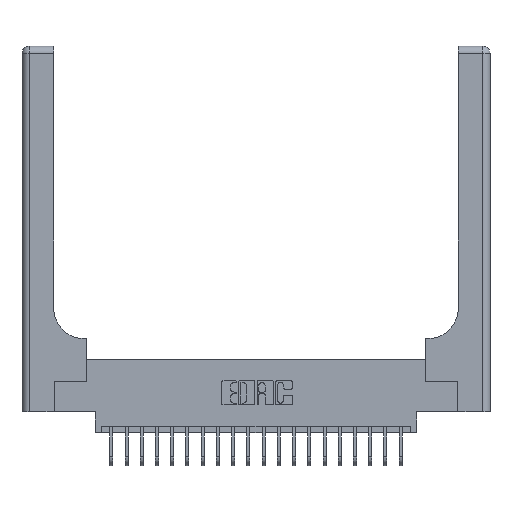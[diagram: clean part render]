
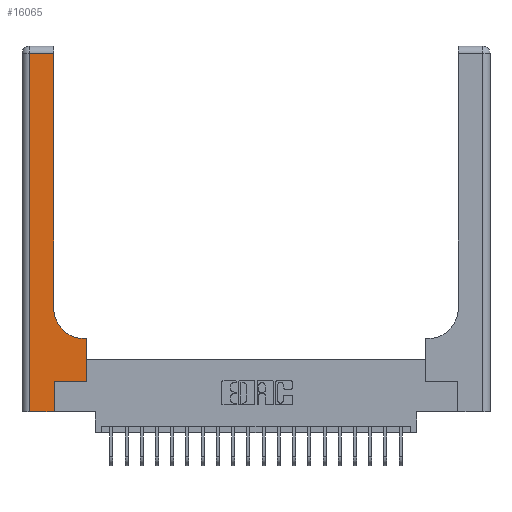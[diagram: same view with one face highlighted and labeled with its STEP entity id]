
A CAD part, top view. The second image highlights one B-rep face of the part: STEP entity #16065.
In plain terms, the highlighted planar face has unit normal (0, 0, 1).
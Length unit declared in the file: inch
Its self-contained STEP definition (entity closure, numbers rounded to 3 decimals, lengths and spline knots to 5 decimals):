
#262 = ORIENTED_EDGE ( 'NONE', *, *, #10968, .T. ) ;
#756 = ORIENTED_EDGE ( 'NONE', *, *, #4540, .T. ) ;
#783 = CARTESIAN_POINT ( 'NONE',  ( 0.528, 0.25, 0.37 ) ) ;
#866 = EDGE_CURVE ( 'NONE', #3148, #17993, #5105, .T. ) ;
#1039 = CARTESIAN_POINT ( 'NONE',  ( 0.265, 0.25, 0.37 ) ) ;
#1550 = VERTEX_POINT ( 'NONE', #18192 ) ;
#2073 = CARTESIAN_POINT ( 'NONE',  ( 0.51, 0.85, 0.37 ) ) ;
#2515 = AXIS2_PLACEMENT_3D ( 'NONE', #2073, #13334, #3703 ) ;
#2525 = CARTESIAN_POINT ( 'NONE',  ( 0.26, 0.6, 0.37 ) ) ;
#2943 = DIRECTION ( 'NONE',  ( -1., 0., 0. ) ) ;
#3007 = AXIS2_PLACEMENT_3D ( 'NONE', #17325, #12579, #2943 ) ;
#3048 = ORIENTED_EDGE ( 'NONE', *, *, #19050, .T. ) ;
#3148 = VERTEX_POINT ( 'NONE', #5501 ) ;
#3211 = EDGE_CURVE ( 'NONE', #4717, #1550, #7536, .T. ) ;
#3476 = VECTOR ( 'NONE', #15523, 39.37008 ) ;
#3703 = DIRECTION ( 'NONE',  ( 1., 0., 0. ) ) ;
#4015 = CARTESIAN_POINT ( 'NONE',  ( 0., 2.94, 0.37 ) ) ;
#4189 = CARTESIAN_POINT ( 'NONE',  ( 0.26, 3., 0.37 ) ) ;
#4418 = CARTESIAN_POINT ( 'NONE',  ( 0.265, 0., 0.37 ) ) ;
#4540 = EDGE_CURVE ( 'NONE', #6452, #16819, #16976, .T. ) ;
#4542 = CARTESIAN_POINT ( 'NONE',  ( 0.26, 2.94, 0.37 ) ) ;
#4717 = VERTEX_POINT ( 'NONE', #4542 ) ;
#5105 = LINE ( 'NONE', #16107, #17397 ) ;
#5501 = CARTESIAN_POINT ( 'NONE',  ( 0.06, 0., 0.37 ) ) ;
#5580 = ORIENTED_EDGE ( 'NONE', *, *, #14114, .T. ) ;
#5660 = VERTEX_POINT ( 'NONE', #17968 ) ;
#5806 = DIRECTION ( 'NONE',  ( 0., 1., 0. ) ) ;
#5862 = LINE ( 'NONE', #2525, #10161 ) ;
#5898 = CARTESIAN_POINT ( 'NONE',  ( 0.265, 0.25, 0.37 ) ) ;
#6035 = DIRECTION ( 'NONE',  ( 0., 1., 0. ) ) ;
#6452 = VERTEX_POINT ( 'NONE', #7565 ) ;
#6500 = DIRECTION ( 'NONE',  ( 1., 0., 0. ) ) ;
#7536 = LINE ( 'NONE', #4015, #14569 ) ;
#7565 = CARTESIAN_POINT ( 'NONE',  ( 0.528, 0.25, 0.37 ) ) ;
#7762 = LINE ( 'NONE', #5898, #3476 ) ;
#7835 = CARTESIAN_POINT ( 'NONE',  ( 0.26, 0.85, 0.37 ) ) ;
#8107 = CARTESIAN_POINT ( 'NONE',  ( 0.06, 3., 0.37 ) ) ;
#8207 = EDGE_CURVE ( 'NONE', #5660, #9135, #14369, .T. ) ;
#8454 = EDGE_CURVE ( 'NONE', #9135, #4717, #13604, .T. ) ;
#8461 = VECTOR ( 'NONE', #19999, 39.37008 ) ;
#9135 = VERTEX_POINT ( 'NONE', #7835 ) ;
#9410 = VECTOR ( 'NONE', #14565, 39.37008 ) ;
#9501 = CARTESIAN_POINT ( 'NONE',  ( 0.265, 0., 0.37 ) ) ;
#9694 = CARTESIAN_POINT ( 'NONE',  ( 0.528, 0.6, 0.37 ) ) ;
#10161 = VECTOR ( 'NONE', #15399, 39.37008 ) ;
#10968 = EDGE_CURVE ( 'NONE', #17200, #6452, #7762, .T. ) ;
#10985 = PLANE ( 'NONE',  #3007 ) ;
#11021 = EDGE_CURVE ( 'NONE', #17993, #17200, #19517, .T. ) ;
#11047 = VECTOR ( 'NONE', #6035, 39.37008 ) ;
#11612 = ORIENTED_EDGE ( 'NONE', *, *, #866, .T. ) ;
#12579 = DIRECTION ( 'NONE',  ( 0., 0., -1. ) ) ;
#12823 = FACE_OUTER_BOUND ( 'NONE', #16762, .T. ) ;
#13334 = DIRECTION ( 'NONE',  ( 0., 0., -1. ) ) ;
#13604 = LINE ( 'NONE', #4189, #17332 ) ;
#13672 = LINE ( 'NONE', #8107, #9410 ) ;
#14114 = EDGE_CURVE ( 'NONE', #16819, #5660, #5862, .T. ) ;
#14369 = CIRCLE ( 'NONE', #2515, 0.25 ) ;
#14565 = DIRECTION ( 'NONE',  ( 0., -1., 0. ) ) ;
#14569 = VECTOR ( 'NONE', #20034, 39.37008 ) ;
#15380 = ORIENTED_EDGE ( 'NONE', *, *, #8454, .T. ) ;
#15399 = DIRECTION ( 'NONE',  ( -1., 0., 0. ) ) ;
#15523 = DIRECTION ( 'NONE',  ( 1., 0., 0. ) ) ;
#16065 = ADVANCED_FACE ( 'NONE', ( #12823 ), #10985, .F. ) ;
#16107 = CARTESIAN_POINT ( 'NONE',  ( 0., 0., 0.37 ) ) ;
#16373 = ORIENTED_EDGE ( 'NONE', *, *, #11021, .T. ) ;
#16762 = EDGE_LOOP ( 'NONE', ( #15380, #19595, #3048, #11612, #16373, #262, #756, #5580, #18374 ) ) ;
#16819 = VERTEX_POINT ( 'NONE', #9694 ) ;
#16976 = LINE ( 'NONE', #783, #8461 ) ;
#17200 = VERTEX_POINT ( 'NONE', #1039 ) ;
#17325 = CARTESIAN_POINT ( 'NONE',  ( 0., 3., 0.37 ) ) ;
#17332 = VECTOR ( 'NONE', #5806, 39.37008 ) ;
#17397 = VECTOR ( 'NONE', #6500, 39.37008 ) ;
#17968 = CARTESIAN_POINT ( 'NONE',  ( 0.51, 0.6, 0.37 ) ) ;
#17993 = VERTEX_POINT ( 'NONE', #9501 ) ;
#18192 = CARTESIAN_POINT ( 'NONE',  ( 0.06, 2.94, 0.37 ) ) ;
#18374 = ORIENTED_EDGE ( 'NONE', *, *, #8207, .T. ) ;
#19050 = EDGE_CURVE ( 'NONE', #1550, #3148, #13672, .T. ) ;
#19517 = LINE ( 'NONE', #4418, #11047 ) ;
#19595 = ORIENTED_EDGE ( 'NONE', *, *, #3211, .T. ) ;
#19999 = DIRECTION ( 'NONE',  ( 0., 1., 0. ) ) ;
#20034 = DIRECTION ( 'NONE',  ( -1., 0., 0. ) ) ;
